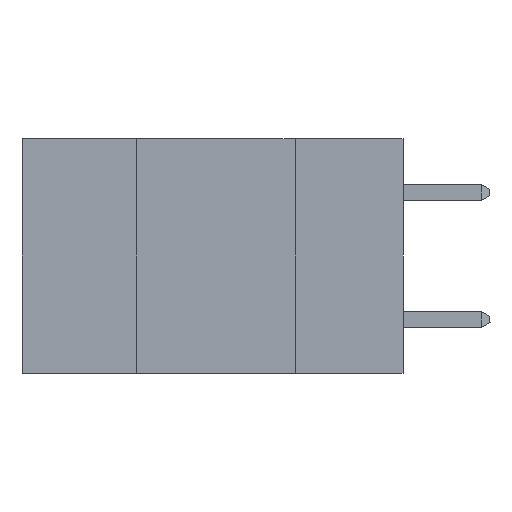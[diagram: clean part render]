
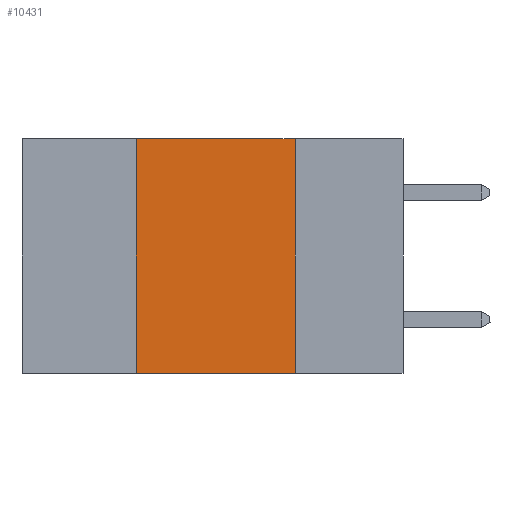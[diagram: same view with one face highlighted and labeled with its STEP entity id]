
A CAD part, left-side view. The second image highlights one B-rep face of the part: STEP entity #10431.
In plain terms, the highlighted planar face has unit normal (-1, 0, 0).
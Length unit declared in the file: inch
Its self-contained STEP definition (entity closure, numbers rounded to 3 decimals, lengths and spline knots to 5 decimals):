
#1006 = LINE ( 'NONE', #9825, #18493 ) ;
#1307 = VECTOR ( 'NONE', #11731, 39.37008 ) ;
#1438 = VECTOR ( 'NONE', #4541, 39.37008 ) ;
#1754 = EDGE_LOOP ( 'NONE', ( #6338, #10776, #20196, #7383 ) ) ;
#2183 = PLANE ( 'NONE',  #13850 ) ;
#2426 = CARTESIAN_POINT ( 'NONE',  ( 0., 0.17, -0.37 ) ) ;
#3389 = CARTESIAN_POINT ( 'NONE',  ( 0., 0.42, 0. ) ) ;
#3520 = CARTESIAN_POINT ( 'NONE',  ( 0., 0.17, 0. ) ) ;
#4097 = CARTESIAN_POINT ( 'NONE',  ( 0., 0.6, -0.37 ) ) ;
#4165 = VECTOR ( 'NONE', #5784, 39.37008 ) ;
#4541 = DIRECTION ( 'NONE',  ( 0., 0., -1. ) ) ;
#4693 = CARTESIAN_POINT ( 'NONE',  ( 0., 0.42, 0. ) ) ;
#5784 = DIRECTION ( 'NONE',  ( 0., -1., 0. ) ) ;
#6338 = ORIENTED_EDGE ( 'NONE', *, *, #19120, .F. ) ;
#6462 = LINE ( 'NONE', #3389, #1307 ) ;
#6992 = FACE_OUTER_BOUND ( 'NONE', #1754, .T. ) ;
#7324 = DIRECTION ( 'NONE',  ( 1., 0., 0. ) ) ;
#7383 = ORIENTED_EDGE ( 'NONE', *, *, #8572, .T. ) ;
#8357 = VERTEX_POINT ( 'NONE', #3520 ) ;
#8572 = EDGE_CURVE ( 'NONE', #13127, #12122, #13090, .T. ) ;
#9825 = CARTESIAN_POINT ( 'NONE',  ( 0., 0.6, 0. ) ) ;
#9896 = DIRECTION ( 'NONE',  ( 0., -1., 0. ) ) ;
#9943 = LINE ( 'NONE', #14689, #1438 ) ;
#10431 = ADVANCED_FACE ( 'NONE', ( #6992 ), #2183, .F. ) ;
#10776 = ORIENTED_EDGE ( 'NONE', *, *, #11210, .F. ) ;
#11210 = EDGE_CURVE ( 'NONE', #12320, #8357, #1006, .T. ) ;
#11731 = DIRECTION ( 'NONE',  ( 0., 0., 1. ) ) ;
#12122 = VERTEX_POINT ( 'NONE', #2426 ) ;
#12320 = VERTEX_POINT ( 'NONE', #4693 ) ;
#13090 = LINE ( 'NONE', #4097, #4165 ) ;
#13127 = VERTEX_POINT ( 'NONE', #15092 ) ;
#13850 = AXIS2_PLACEMENT_3D ( 'NONE', #17387, #7324, #19030 ) ;
#14689 = CARTESIAN_POINT ( 'NONE',  ( 0., 0.17, 0. ) ) ;
#15092 = CARTESIAN_POINT ( 'NONE',  ( 0., 0.42, -0.37 ) ) ;
#15790 = EDGE_CURVE ( 'NONE', #13127, #12320, #6462, .T. ) ;
#17387 = CARTESIAN_POINT ( 'NONE',  ( 0., 0.6, 0. ) ) ;
#18493 = VECTOR ( 'NONE', #9896, 39.37008 ) ;
#19030 = DIRECTION ( 'NONE',  ( 0., 0., -1. ) ) ;
#19120 = EDGE_CURVE ( 'NONE', #8357, #12122, #9943, .T. ) ;
#20196 = ORIENTED_EDGE ( 'NONE', *, *, #15790, .F. ) ;
